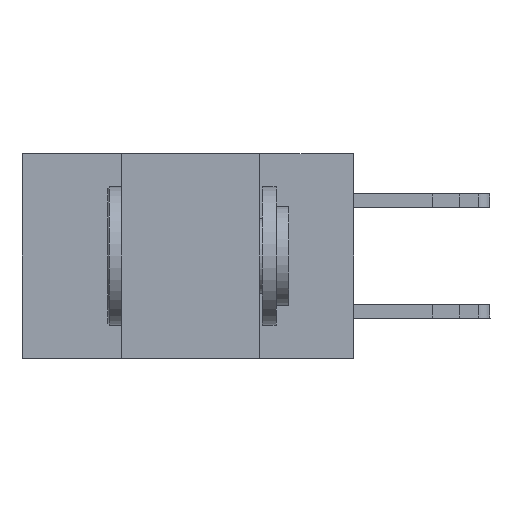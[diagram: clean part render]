
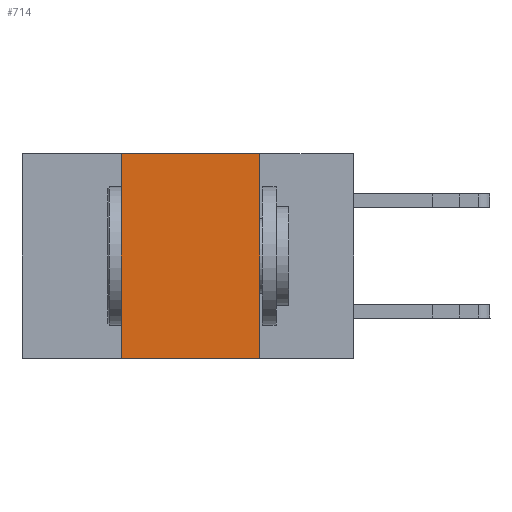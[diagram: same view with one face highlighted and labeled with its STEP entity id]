
A CAD part, left-side view. The second image highlights one B-rep face of the part: STEP entity #714.
In plain terms, the highlighted planar face has unit normal (-1, 0, 0).
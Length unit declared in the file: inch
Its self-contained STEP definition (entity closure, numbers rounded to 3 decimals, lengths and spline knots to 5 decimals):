
#610 = CARTESIAN_POINT ( 'NONE',  ( 0., 0.42, -0.37 ) ) ;
#714 = ADVANCED_FACE ( 'NONE', ( #1164 ), #10420, .F. ) ;
#1164 = FACE_OUTER_BOUND ( 'NONE', #6646, .T. ) ;
#1356 = EDGE_CURVE ( 'NONE', #18940, #20238, #13194, .T. ) ;
#1763 = CARTESIAN_POINT ( 'NONE',  ( 0., 0.6, 0. ) ) ;
#2871 = CARTESIAN_POINT ( 'NONE',  ( 0., 0.6, -0.37 ) ) ;
#3413 = DIRECTION ( 'NONE',  ( 0., 0., -1. ) ) ;
#3417 = VECTOR ( 'NONE', #18075, 39.37008 ) ;
#3768 = LINE ( 'NONE', #17748, #20623 ) ;
#6646 = EDGE_LOOP ( 'NONE', ( #21721, #12635, #7560, #11867 ) ) ;
#7124 = DIRECTION ( 'NONE',  ( 1., 0., 0. ) ) ;
#7220 = DIRECTION ( 'NONE',  ( 0., 0., -1. ) ) ;
#7560 = ORIENTED_EDGE ( 'NONE', *, *, #17557, .F. ) ;
#7947 = CARTESIAN_POINT ( 'NONE',  ( 0., 0.42, 0. ) ) ;
#8449 = LINE ( 'NONE', #13625, #18397 ) ;
#9734 = VERTEX_POINT ( 'NONE', #14023 ) ;
#10420 = PLANE ( 'NONE',  #12349 ) ;
#11867 = ORIENTED_EDGE ( 'NONE', *, *, #1356, .T. ) ;
#12349 = AXIS2_PLACEMENT_3D ( 'NONE', #1763, #7124, #7220 ) ;
#12578 = DIRECTION ( 'NONE',  ( 0., 0., 1. ) ) ;
#12635 = ORIENTED_EDGE ( 'NONE', *, *, #17560, .F. ) ;
#13019 = CARTESIAN_POINT ( 'NONE',  ( 0., 0.17, -0.37 ) ) ;
#13155 = VECTOR ( 'NONE', #22095, 39.37008 ) ;
#13194 = LINE ( 'NONE', #2871, #13155 ) ;
#13625 = CARTESIAN_POINT ( 'NONE',  ( 0., 0.17, 0. ) ) ;
#14023 = CARTESIAN_POINT ( 'NONE',  ( 0., 0.17, 0. ) ) ;
#16027 = EDGE_CURVE ( 'NONE', #9734, #20238, #8449, .T. ) ;
#16364 = LINE ( 'NONE', #21279, #3417 ) ;
#17557 = EDGE_CURVE ( 'NONE', #18940, #20671, #3768, .T. ) ;
#17560 = EDGE_CURVE ( 'NONE', #20671, #9734, #16364, .T. ) ;
#17748 = CARTESIAN_POINT ( 'NONE',  ( 0., 0.42, 0. ) ) ;
#18075 = DIRECTION ( 'NONE',  ( 0., -1., 0. ) ) ;
#18397 = VECTOR ( 'NONE', #3413, 39.37008 ) ;
#18940 = VERTEX_POINT ( 'NONE', #610 ) ;
#20238 = VERTEX_POINT ( 'NONE', #13019 ) ;
#20623 = VECTOR ( 'NONE', #12578, 39.37008 ) ;
#20671 = VERTEX_POINT ( 'NONE', #7947 ) ;
#21279 = CARTESIAN_POINT ( 'NONE',  ( 0., 0.6, 0. ) ) ;
#21721 = ORIENTED_EDGE ( 'NONE', *, *, #16027, .F. ) ;
#22095 = DIRECTION ( 'NONE',  ( 0., -1., 0. ) ) ;
